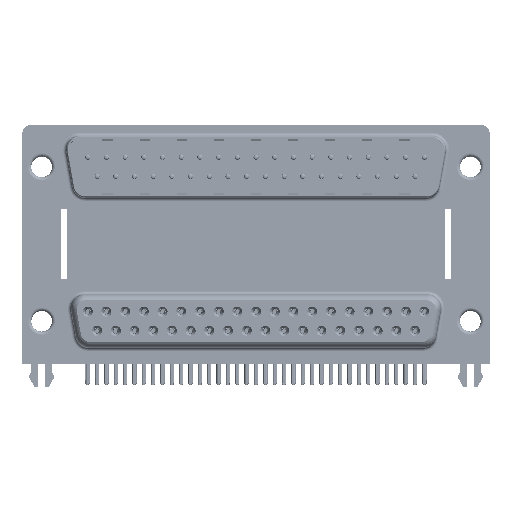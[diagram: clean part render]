
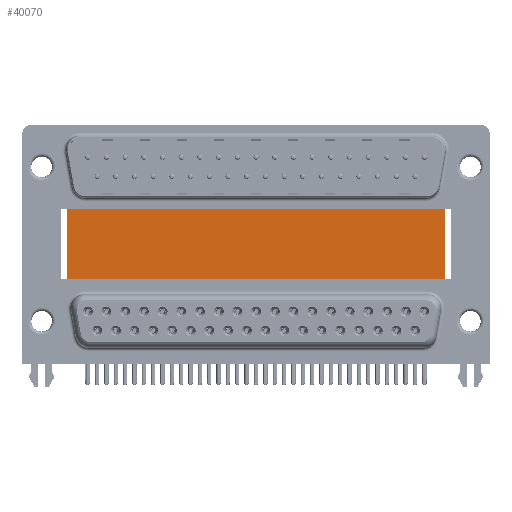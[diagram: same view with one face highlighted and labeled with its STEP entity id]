
A CAD part, top view. The second image highlights one B-rep face of the part: STEP entity #40070.
In plain terms, the highlighted planar face has unit normal (0, 0, 1).
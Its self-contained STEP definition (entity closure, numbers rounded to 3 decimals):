
#1178 = CARTESIAN_POINT ( 'NONE',  ( 3.79, 16.585, -12. ) ) ;
#3608 = EDGE_CURVE ( 'NONE', #63006, #8742, #17612, .T. ) ;
#5780 = VERTEX_POINT ( 'NONE', #59427 ) ;
#8742 = VERTEX_POINT ( 'NONE', #21882 ) ;
#11618 = DIRECTION ( 'NONE',  ( 0., 0., -1. ) ) ;
#12362 = VECTOR ( 'NONE', #64037, 1000. ) ;
#17089 = AXIS2_PLACEMENT_3D ( 'NONE', #18084, #11618, #22585 ) ;
#17612 = LINE ( 'NONE', #38576, #65029 ) ;
#18084 = CARTESIAN_POINT ( 'NONE',  ( 3.79, 16.585, -12. ) ) ;
#21882 = CARTESIAN_POINT ( 'NONE',  ( 59.71, 16.585, -12. ) ) ;
#22585 = DIRECTION ( 'NONE',  ( -1., 0., 0. ) ) ;
#23149 = ORIENTED_EDGE ( 'NONE', *, *, #29852, .T. ) ;
#23155 = ORIENTED_EDGE ( 'NONE', *, *, #3608, .F. ) ;
#25913 = DIRECTION ( 'NONE',  ( 0., -1., 0. ) ) ;
#26299 = VECTOR ( 'NONE', #58322, 1000. ) ;
#26603 = CARTESIAN_POINT ( 'NONE',  ( 59.71, 16.585, -12. ) ) ;
#28003 = CARTESIAN_POINT ( 'NONE',  ( 3.79, 16.585, -12. ) ) ;
#28278 = LINE ( 'NONE', #1178, #12362 ) ;
#29852 = EDGE_CURVE ( 'NONE', #66448, #5780, #52156, .T. ) ;
#37404 = CARTESIAN_POINT ( 'NONE',  ( 3.79, -3.735, -12. ) ) ;
#38576 = CARTESIAN_POINT ( 'NONE',  ( 3.79, 16.585, -12. ) ) ;
#40070 = ADVANCED_FACE ( 'NONE', ( #43208 ), #44206, .F. ) ;
#42406 = LINE ( 'NONE', #26603, #55665 ) ;
#42471 = CARTESIAN_POINT ( 'NONE',  ( 3.79, -3.735, -12. ) ) ;
#43208 = FACE_OUTER_BOUND ( 'NONE', #61763, .T. ) ;
#44206 = PLANE ( 'NONE',  #17089 ) ;
#52156 = LINE ( 'NONE', #37404, #26299 ) ;
#52781 = EDGE_CURVE ( 'NONE', #63006, #66448, #28278, .T. ) ;
#55665 = VECTOR ( 'NONE', #25913, 1000. ) ;
#56169 = ORIENTED_EDGE ( 'NONE', *, *, #52781, .T. ) ;
#57433 = EDGE_CURVE ( 'NONE', #8742, #5780, #42406, .T. ) ;
#58322 = DIRECTION ( 'NONE',  ( 1., 0., 0. ) ) ;
#59427 = CARTESIAN_POINT ( 'NONE',  ( 59.71, -3.735, -12. ) ) ;
#59510 = DIRECTION ( 'NONE',  ( 1., 0., 0. ) ) ;
#61763 = EDGE_LOOP ( 'NONE', ( #23149, #66878, #23155, #56169 ) ) ;
#63006 = VERTEX_POINT ( 'NONE', #28003 ) ;
#64037 = DIRECTION ( 'NONE',  ( 0., -1., 0. ) ) ;
#65029 = VECTOR ( 'NONE', #59510, 1000. ) ;
#66448 = VERTEX_POINT ( 'NONE', #42471 ) ;
#66878 = ORIENTED_EDGE ( 'NONE', *, *, #57433, .F. ) ;
